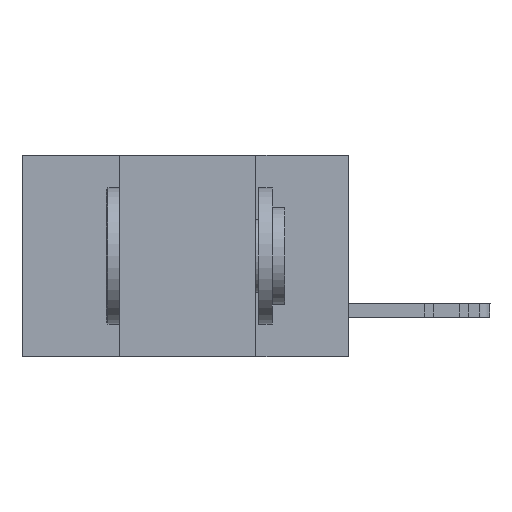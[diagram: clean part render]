
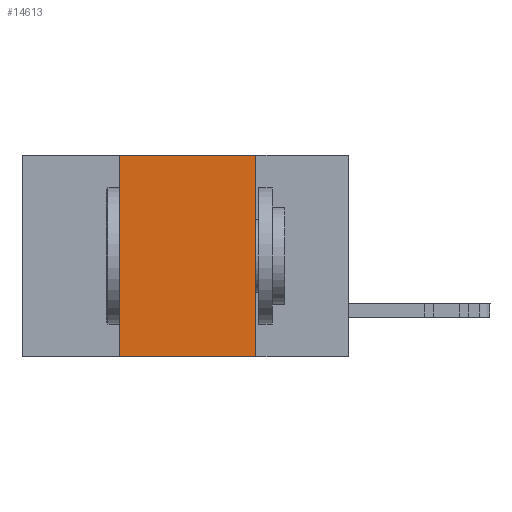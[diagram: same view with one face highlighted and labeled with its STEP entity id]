
A CAD part, left-side view. The second image highlights one B-rep face of the part: STEP entity #14613.
In plain terms, the highlighted planar face has unit normal (-1, 0, 0).
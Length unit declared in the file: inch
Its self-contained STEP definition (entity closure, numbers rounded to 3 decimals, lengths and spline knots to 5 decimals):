
#75 = CARTESIAN_POINT ( 'NONE',  ( 0., 0.17, 0. ) ) ;
#524 = CARTESIAN_POINT ( 'NONE',  ( 0., 0.42, -0.37 ) ) ;
#769 = DIRECTION ( 'NONE',  ( 0., 0., -1. ) ) ;
#1160 = DIRECTION ( 'NONE',  ( 0., -1., 0. ) ) ;
#1313 = ORIENTED_EDGE ( 'NONE', *, *, #16546, .T. ) ;
#1372 = DIRECTION ( 'NONE',  ( 0., -1., 0. ) ) ;
#5260 = CARTESIAN_POINT ( 'NONE',  ( 0., 0.17, -0.37 ) ) ;
#5383 = AXIS2_PLACEMENT_3D ( 'NONE', #16732, #20165, #24445 ) ;
#6598 = CARTESIAN_POINT ( 'NONE',  ( 0., 0.17, -0.37 ) ) ;
#7026 = FACE_OUTER_BOUND ( 'NONE', #12718, .T. ) ;
#8212 = VECTOR ( 'NONE', #1372, 39.37008 ) ;
#8366 = VECTOR ( 'NONE', #769, 39.37008 ) ;
#8877 = LINE ( 'NONE', #18708, #9311 ) ;
#9311 = VECTOR ( 'NONE', #1160, 39.37008 ) ;
#9649 = DIRECTION ( 'NONE',  ( 0., 0., 1. ) ) ;
#10958 = ORIENTED_EDGE ( 'NONE', *, *, #15298, .F. ) ;
#11568 = EDGE_CURVE ( 'NONE', #24051, #14837, #8877, .T. ) ;
#11595 = CARTESIAN_POINT ( 'NONE',  ( 0., 0.42, 0. ) ) ;
#12718 = EDGE_LOOP ( 'NONE', ( #21895, #21460, #10958, #1313 ) ) ;
#13387 = VERTEX_POINT ( 'NONE', #5260 ) ;
#14613 = ADVANCED_FACE ( 'NONE', ( #7026 ), #20527, .F. ) ;
#14837 = VERTEX_POINT ( 'NONE', #75 ) ;
#14894 = LINE ( 'NONE', #20578, #8212 ) ;
#15298 = EDGE_CURVE ( 'NONE', #20729, #24051, #19228, .T. ) ;
#16546 = EDGE_CURVE ( 'NONE', #20729, #13387, #14894, .T. ) ;
#16732 = CARTESIAN_POINT ( 'NONE',  ( 0., 0.6, 0. ) ) ;
#17828 = VECTOR ( 'NONE', #9649, 39.37008 ) ;
#18708 = CARTESIAN_POINT ( 'NONE',  ( 0., 0.6, 0. ) ) ;
#19228 = LINE ( 'NONE', #21253, #17828 ) ;
#20165 = DIRECTION ( 'NONE',  ( 1., 0., 0. ) ) ;
#20527 = PLANE ( 'NONE',  #5383 ) ;
#20578 = CARTESIAN_POINT ( 'NONE',  ( 0., 0.6, -0.37 ) ) ;
#20704 = EDGE_CURVE ( 'NONE', #14837, #13387, #21614, .T. ) ;
#20729 = VERTEX_POINT ( 'NONE', #524 ) ;
#21253 = CARTESIAN_POINT ( 'NONE',  ( 0., 0.42, -0.37 ) ) ;
#21460 = ORIENTED_EDGE ( 'NONE', *, *, #11568, .F. ) ;
#21614 = LINE ( 'NONE', #6598, #8366 ) ;
#21895 = ORIENTED_EDGE ( 'NONE', *, *, #20704, .F. ) ;
#24051 = VERTEX_POINT ( 'NONE', #11595 ) ;
#24445 = DIRECTION ( 'NONE',  ( 0., 0., -1. ) ) ;
